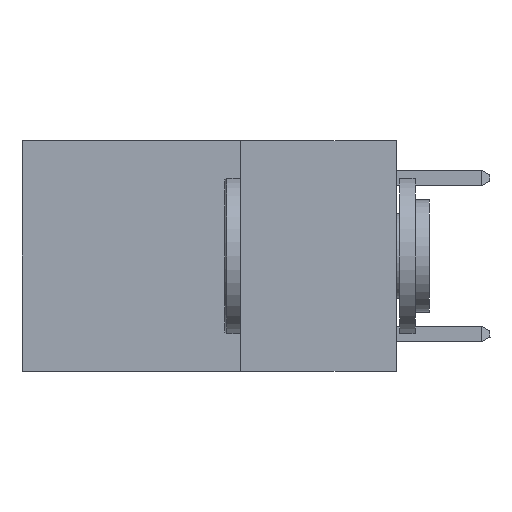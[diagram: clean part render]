
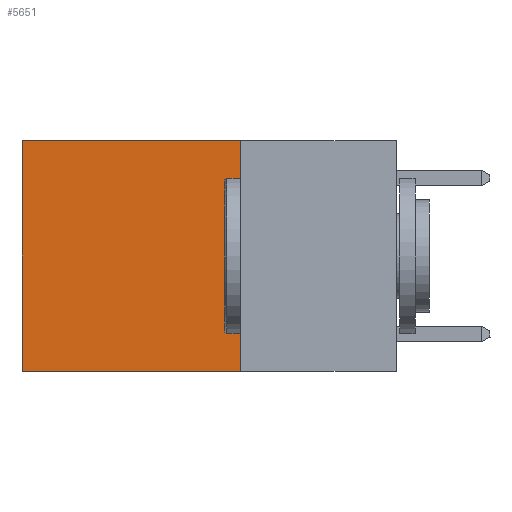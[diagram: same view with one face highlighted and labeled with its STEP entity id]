
A CAD part, left-side view. The second image highlights one B-rep face of the part: STEP entity #5651.
In plain terms, the highlighted planar face has unit normal (-1, 0, 0).
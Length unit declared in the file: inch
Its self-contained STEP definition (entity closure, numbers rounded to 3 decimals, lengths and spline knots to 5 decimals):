
#72 = VECTOR ( 'NONE', #3247, 39.37008 ) ;
#286 = EDGE_LOOP ( 'NONE', ( #6490, #1525, #5388, #10577 ) ) ;
#507 = CARTESIAN_POINT ( 'NONE',  ( 0.2625, 0.25, -0.37 ) ) ;
#606 = CARTESIAN_POINT ( 'NONE',  ( 0.2625, 0.25, 0. ) ) ;
#769 = CARTESIAN_POINT ( 'NONE',  ( 0.2625, 0.25, 0. ) ) ;
#955 = DIRECTION ( 'NONE',  ( 0., 0., -1. ) ) ;
#1276 = LINE ( 'NONE', #606, #3806 ) ;
#1525 = ORIENTED_EDGE ( 'NONE', *, *, #10846, .F. ) ;
#2057 = CARTESIAN_POINT ( 'NONE',  ( 0.2625, 0.6, 0. ) ) ;
#2599 = CARTESIAN_POINT ( 'NONE',  ( 0.2625, 0.25, -0.37 ) ) ;
#2642 = DIRECTION ( 'NONE',  ( 0., 1., 0. ) ) ;
#3167 = VECTOR ( 'NONE', #955, 39.37008 ) ;
#3247 = DIRECTION ( 'NONE',  ( 0., 1., 0. ) ) ;
#3290 = DIRECTION ( 'NONE',  ( 1., 0., 0. ) ) ;
#3806 = VECTOR ( 'NONE', #5940, 39.37008 ) ;
#4571 = VERTEX_POINT ( 'NONE', #769 ) ;
#4806 = VECTOR ( 'NONE', #2642, 39.37008 ) ;
#4821 = VERTEX_POINT ( 'NONE', #9312 ) ;
#5388 = ORIENTED_EDGE ( 'NONE', *, *, #10927, .F. ) ;
#5519 = FACE_OUTER_BOUND ( 'NONE', #286, .T. ) ;
#5651 = ADVANCED_FACE ( 'NONE', ( #5519 ), #9615, .F. ) ;
#5652 = AXIS2_PLACEMENT_3D ( 'NONE', #12572, #3290, #10614 ) ;
#5940 = DIRECTION ( 'NONE',  ( 0., 0., -1. ) ) ;
#5980 = LINE ( 'NONE', #2057, #3167 ) ;
#6490 = ORIENTED_EDGE ( 'NONE', *, *, #6769, .T. ) ;
#6769 = EDGE_CURVE ( 'NONE', #4821, #6906, #5980, .T. ) ;
#6906 = VERTEX_POINT ( 'NONE', #7556 ) ;
#7455 = CARTESIAN_POINT ( 'NONE',  ( 0.2625, 0.25, 0. ) ) ;
#7508 = EDGE_CURVE ( 'NONE', #4571, #4821, #8586, .T. ) ;
#7556 = CARTESIAN_POINT ( 'NONE',  ( 0.2625, 0.6, -0.37 ) ) ;
#8586 = LINE ( 'NONE', #7455, #72 ) ;
#9312 = CARTESIAN_POINT ( 'NONE',  ( 0.2625, 0.6, 0. ) ) ;
#9615 = PLANE ( 'NONE',  #5652 ) ;
#10371 = LINE ( 'NONE', #2599, #4806 ) ;
#10577 = ORIENTED_EDGE ( 'NONE', *, *, #7508, .T. ) ;
#10614 = DIRECTION ( 'NONE',  ( 0., 0., -1. ) ) ;
#10846 = EDGE_CURVE ( 'NONE', #10871, #6906, #10371, .T. ) ;
#10871 = VERTEX_POINT ( 'NONE', #507 ) ;
#10927 = EDGE_CURVE ( 'NONE', #4571, #10871, #1276, .T. ) ;
#12572 = CARTESIAN_POINT ( 'NONE',  ( 0.2625, 0.25, 0. ) ) ;
